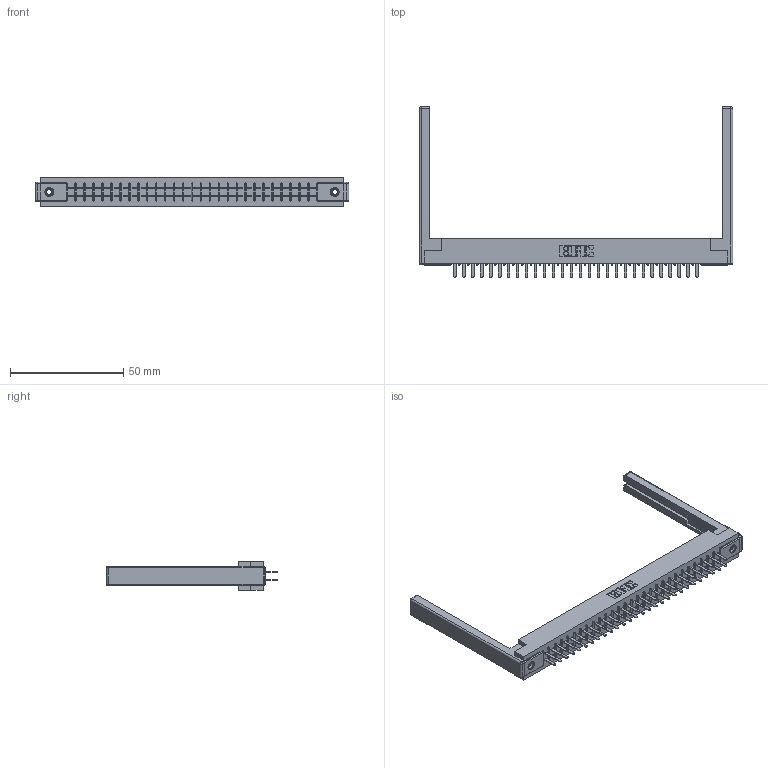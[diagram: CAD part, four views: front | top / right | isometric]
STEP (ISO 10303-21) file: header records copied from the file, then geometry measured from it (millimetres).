
FILE_DESCRIPTION (( 'STEP AP203' ), '1' );
FILE_NAME ('315-056-520-268.STEP', '2019-09-10T19:25:30', ( '' ), ( '' ), 'SwSTEP 2.0', 'SolidWorks 2016', '' );
FILE_SCHEMA (( 'CONFIG_CONTROL_DESIGN' ));
Length unit declared in the file: inch
Products named in the file (5): 315-056-520-268; 345-250-001_345-250-001-102; 305 Part_.156 Dia; 305-290-001_520; 307-220-068
Assembly tree (61 placements, depth 2):
  315-056-520-268
    305 Part_.156 Dia
    305-290-001_520  x56
    345-250-001_345-250-001-102  x2
    307-220-068  x2
Bounding box: 138.38 x 75.39 x 12.7 mm (x, y, z)
Volume: 18741.2 mm3; surface area: 21941.1 mm2
Topology: 61 solids, 61 shells, 2846 faces, 8070 edges, 5208 vertices
Faces by surface type: plane 1668, cylinder 1042, sphere 120, cone 12, torus 4
Entity records: 34660 total; most frequent: CARTESIAN_POINT 5707, ORIENTED_EDGE 5654, DIRECTION 5551, EDGE_CURVE 2827, VECTOR 2263, LINE 2263, VERTEX_POINT 1800, AXIS2_PLACEMENT_3D 1644
